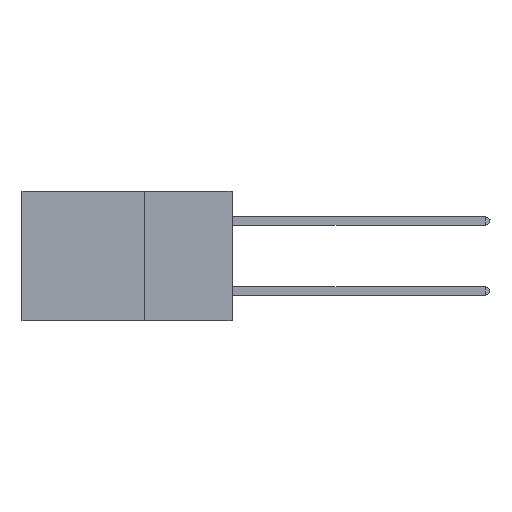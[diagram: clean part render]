
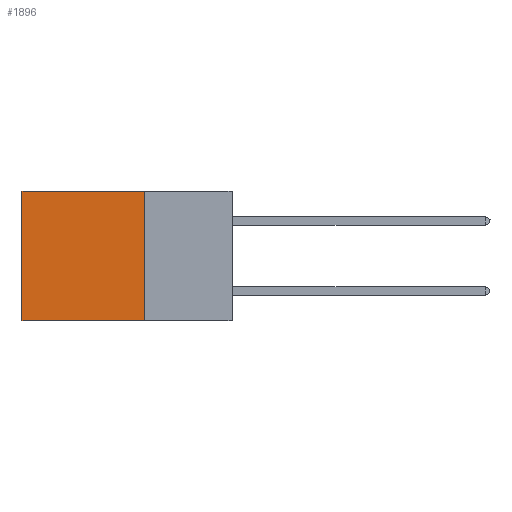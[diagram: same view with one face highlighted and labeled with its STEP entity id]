
A CAD part, left-side view. The second image highlights one B-rep face of the part: STEP entity #1896.
In plain terms, the highlighted planar face has unit normal (-1, 0, 0).
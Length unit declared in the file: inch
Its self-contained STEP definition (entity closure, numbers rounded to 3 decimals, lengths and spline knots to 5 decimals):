
#195 = LINE ( 'NONE', #3236, #6615 ) ;
#1459 = ORIENTED_EDGE ( 'NONE', *, *, #11235, .F. ) ;
#1896 = ADVANCED_FACE ( 'NONE', ( #18327 ), #34273, .F. ) ;
#3236 = CARTESIAN_POINT ( 'NONE',  ( 0.2875, 0.25, 0. ) ) ;
#4250 = EDGE_CURVE ( 'NONE', #33233, #22492, #39210, .T. ) ;
#4364 = CARTESIAN_POINT ( 'NONE',  ( 0.2875, 0.25, 0. ) ) ;
#6615 = VECTOR ( 'NONE', #28191, 39.37008 ) ;
#8588 = LINE ( 'NONE', #4364, #29022 ) ;
#9174 = CARTESIAN_POINT ( 'NONE',  ( 0.2875, 0.25, 0. ) ) ;
#11235 = EDGE_CURVE ( 'NONE', #25358, #33233, #195, .T. ) ;
#11360 = CARTESIAN_POINT ( 'NONE',  ( 0.2875, 0.6, -0.37 ) ) ;
#12264 = EDGE_CURVE ( 'NONE', #34440, #22492, #14099, .T. ) ;
#13124 = VECTOR ( 'NONE', #14869, 39.37008 ) ;
#13999 = AXIS2_PLACEMENT_3D ( 'NONE', #33870, #17925, #24885 ) ;
#14099 = LINE ( 'NONE', #19637, #28645 ) ;
#14869 = DIRECTION ( 'NONE',  ( 0., 1., 0. ) ) ;
#16903 = CARTESIAN_POINT ( 'NONE',  ( 0.2875, 0.6, 0. ) ) ;
#17523 = CARTESIAN_POINT ( 'NONE',  ( 0.2875, 0.25, -0.37 ) ) ;
#17667 = EDGE_CURVE ( 'NONE', #25358, #34440, #8588, .T. ) ;
#17925 = DIRECTION ( 'NONE',  ( 1., 0., 0. ) ) ;
#18229 = ORIENTED_EDGE ( 'NONE', *, *, #12264, .T. ) ;
#18327 = FACE_OUTER_BOUND ( 'NONE', #18523, .T. ) ;
#18523 = EDGE_LOOP ( 'NONE', ( #18229, #32476, #1459, #39173 ) ) ;
#19637 = CARTESIAN_POINT ( 'NONE',  ( 0.2875, 0.6, 0. ) ) ;
#21844 = DIRECTION ( 'NONE',  ( 0., 1., 0. ) ) ;
#22492 = VERTEX_POINT ( 'NONE', #11360 ) ;
#22919 = DIRECTION ( 'NONE',  ( 0., 0., -1. ) ) ;
#24885 = DIRECTION ( 'NONE',  ( 0., 0., -1. ) ) ;
#25358 = VERTEX_POINT ( 'NONE', #9174 ) ;
#28191 = DIRECTION ( 'NONE',  ( 0., 0., -1. ) ) ;
#28645 = VECTOR ( 'NONE', #22919, 39.37008 ) ;
#29022 = VECTOR ( 'NONE', #21844, 39.37008 ) ;
#29183 = CARTESIAN_POINT ( 'NONE',  ( 0.2875, 0.25, -0.37 ) ) ;
#32476 = ORIENTED_EDGE ( 'NONE', *, *, #4250, .F. ) ;
#33233 = VERTEX_POINT ( 'NONE', #29183 ) ;
#33870 = CARTESIAN_POINT ( 'NONE',  ( 0.2875, 0.25, 0. ) ) ;
#34273 = PLANE ( 'NONE',  #13999 ) ;
#34440 = VERTEX_POINT ( 'NONE', #16903 ) ;
#39173 = ORIENTED_EDGE ( 'NONE', *, *, #17667, .T. ) ;
#39210 = LINE ( 'NONE', #17523, #13124 ) ;
